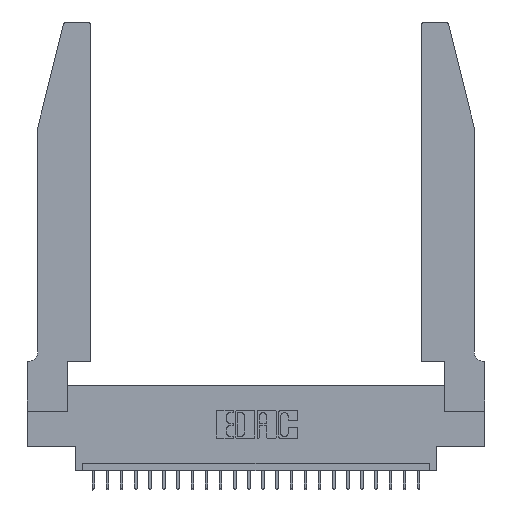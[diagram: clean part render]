
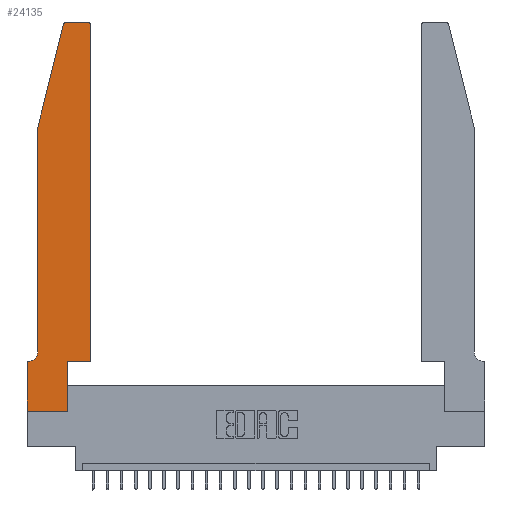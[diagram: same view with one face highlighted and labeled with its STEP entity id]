
A CAD part, top view. The second image highlights one B-rep face of the part: STEP entity #24135.
In plain terms, the highlighted planar face has unit normal (0, 0, 1).
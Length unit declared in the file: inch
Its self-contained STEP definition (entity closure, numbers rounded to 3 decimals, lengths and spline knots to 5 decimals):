
#14 = CARTESIAN_POINT ( 'NONE',  ( 0.4505, 0.35, 0.37 ) ) ;
#51 = AXIS2_PLACEMENT_3D ( 'NONE', #10371, #716, #18200 ) ;
#191 = ORIENTED_EDGE ( 'NONE', *, *, #12260, .T. ) ;
#641 = LINE ( 'NONE', #16233, #10763 ) ;
#716 = DIRECTION ( 'NONE',  ( 0., 0., 1. ) ) ;
#1114 = PLANE ( 'NONE',  #5578 ) ;
#1392 = CARTESIAN_POINT ( 'NONE',  ( 0.0755, 0.35, 0.37 ) ) ;
#1571 = VERTEX_POINT ( 'NONE', #12350 ) ;
#2977 = CARTESIAN_POINT ( 'NONE',  ( 0.0755, 2., 0.37 ) ) ;
#3341 = CARTESIAN_POINT ( 'NONE',  ( 0.0055, 0.42, 0.37 ) ) ;
#3713 = DIRECTION ( 'NONE',  ( -1., 0., 0. ) ) ;
#4016 = ORIENTED_EDGE ( 'NONE', *, *, #24221, .T. ) ;
#4251 = CARTESIAN_POINT ( 'NONE',  ( 0.0755, 2., 0.37 ) ) ;
#4422 = EDGE_CURVE ( 'NONE', #24892, #13779, #7336, .T. ) ;
#4472 = EDGE_CURVE ( 'NONE', #12103, #1571, #8164, .T. ) ;
#5578 = AXIS2_PLACEMENT_3D ( 'NONE', #16710, #6693, #14515 ) ;
#5741 = ORIENTED_EDGE ( 'NONE', *, *, #10918, .T. ) ;
#6001 = CARTESIAN_POINT ( 'NONE',  ( 0.4205, 2.75, 0.37 ) ) ;
#6155 = CARTESIAN_POINT ( 'NONE',  ( 0.2865, 0., 0.37 ) ) ;
#6693 = DIRECTION ( 'NONE',  ( 0., 0., 1. ) ) ;
#6785 = CARTESIAN_POINT ( 'NONE',  ( 0.4505, 0.35, 0.37 ) ) ;
#7231 = DIRECTION ( 'NONE',  ( 0., 1., 0. ) ) ;
#7336 = CIRCLE ( 'NONE', #22119, 0.07 ) ;
#7711 = CARTESIAN_POINT ( 'NONE',  ( 0.4505, 2.72, 0.37 ) ) ;
#8164 = CIRCLE ( 'NONE', #14316, 0.03 ) ;
#8237 = VERTEX_POINT ( 'NONE', #14681 ) ;
#8487 = VECTOR ( 'NONE', #16945, 39.37008 ) ;
#8512 = DIRECTION ( 'NONE',  ( 0., -1., 0. ) ) ;
#8934 = DIRECTION ( 'NONE',  ( 0., 0., 1. ) ) ;
#9115 = FACE_OUTER_BOUND ( 'NONE', #23771, .T. ) ;
#9247 = CARTESIAN_POINT ( 'NONE',  ( 0.2605, 2.75, 0.37 ) ) ;
#9579 = VECTOR ( 'NONE', #3713, 39.37008 ) ;
#9839 = LINE ( 'NONE', #14, #10382 ) ;
#10145 = ORIENTED_EDGE ( 'NONE', *, *, #25281, .T. ) ;
#10371 = CARTESIAN_POINT ( 'NONE',  ( 0.4205, 2.72, 0.37 ) ) ;
#10382 = VECTOR ( 'NONE', #17653, 39.37008 ) ;
#10714 = LINE ( 'NONE', #2977, #22057 ) ;
#10716 = VERTEX_POINT ( 'NONE', #6001 ) ;
#10763 = VECTOR ( 'NONE', #8512, 39.37008 ) ;
#10916 = VECTOR ( 'NONE', #15660, 39.37008 ) ;
#10918 = EDGE_CURVE ( 'NONE', #21798, #10716, #20173, .T. ) ;
#11150 = LINE ( 'NONE', #9247, #20796 ) ;
#11857 = LINE ( 'NONE', #19698, #20212 ) ;
#12103 = VERTEX_POINT ( 'NONE', #17873 ) ;
#12260 = EDGE_CURVE ( 'NONE', #17169, #13302, #641, .T. ) ;
#12350 = CARTESIAN_POINT ( 'NONE',  ( 0.25487, 2.72718, 0.37 ) ) ;
#13122 = VERTEX_POINT ( 'NONE', #24740 ) ;
#13290 = ORIENTED_EDGE ( 'NONE', *, *, #24005, .T. ) ;
#13302 = VERTEX_POINT ( 'NONE', #17529 ) ;
#13452 = ORIENTED_EDGE ( 'NONE', *, *, #4422, .T. ) ;
#13779 = VERTEX_POINT ( 'NONE', #13993 ) ;
#13993 = CARTESIAN_POINT ( 'NONE',  ( 0.0055, 0.35, 0.37 ) ) ;
#14316 = AXIS2_PLACEMENT_3D ( 'NONE', #17143, #8934, #24607 ) ;
#14515 = DIRECTION ( 'NONE',  ( 1., 0., 0. ) ) ;
#14681 = CARTESIAN_POINT ( 'NONE',  ( 0.0755, 2., 0.37 ) ) ;
#14819 = DIRECTION ( 'NONE',  ( -1., 0., 0. ) ) ;
#14838 = CARTESIAN_POINT ( 'NONE',  ( 0., 0.35, 0.37 ) ) ;
#14887 = VECTOR ( 'NONE', #7231, 39.37008 ) ;
#15130 = LINE ( 'NONE', #15531, #10916 ) ;
#15531 = CARTESIAN_POINT ( 'NONE',  ( 0.4505, 0.35, 0.37 ) ) ;
#15660 = DIRECTION ( 'NONE',  ( 0., 1., 0. ) ) ;
#16123 = DIRECTION ( 'NONE',  ( 1., 0., 0. ) ) ;
#16233 = CARTESIAN_POINT ( 'NONE',  ( 0., 0., 0.37 ) ) ;
#16710 = CARTESIAN_POINT ( 'NONE',  ( 0., 0.35, 0.37 ) ) ;
#16945 = DIRECTION ( 'NONE',  ( -0.239, -0.971, 0. ) ) ;
#17143 = CARTESIAN_POINT ( 'NONE',  ( 0.284, 2.72, 0.37 ) ) ;
#17169 = VERTEX_POINT ( 'NONE', #14838 ) ;
#17193 = ORIENTED_EDGE ( 'NONE', *, *, #4472, .T. ) ;
#17529 = CARTESIAN_POINT ( 'NONE',  ( 0., 0., 0.37 ) ) ;
#17653 = DIRECTION ( 'NONE',  ( 1., 0., 0. ) ) ;
#17873 = CARTESIAN_POINT ( 'NONE',  ( 0.284, 2.75, 0.37 ) ) ;
#18200 = DIRECTION ( 'NONE',  ( 1., 0., 0. ) ) ;
#18670 = EDGE_CURVE ( 'NONE', #21903, #13122, #24849, .T. ) ;
#18711 = ORIENTED_EDGE ( 'NONE', *, *, #24792, .T. ) ;
#18784 = CARTESIAN_POINT ( 'NONE',  ( 0.0755, 0.42, 0.37 ) ) ;
#18894 = CARTESIAN_POINT ( 'NONE',  ( 0.2865, 0.35, 0.37 ) ) ;
#18978 = DIRECTION ( 'NONE',  ( -1., 0., 0. ) ) ;
#19200 = VERTEX_POINT ( 'NONE', #6785 ) ;
#19698 = CARTESIAN_POINT ( 'NONE',  ( 0., 0., 0.37 ) ) ;
#19772 = EDGE_CURVE ( 'NONE', #13122, #19200, #9839, .T. ) ;
#19911 = EDGE_CURVE ( 'NONE', #13302, #21903, #11857, .T. ) ;
#20173 = CIRCLE ( 'NONE', #51, 0.03 ) ;
#20212 = VECTOR ( 'NONE', #16123, 39.37008 ) ;
#20252 = EDGE_CURVE ( 'NONE', #13779, #17169, #25220, .T. ) ;
#20796 = VECTOR ( 'NONE', #18978, 39.37008 ) ;
#20840 = DIRECTION ( 'NONE',  ( 0., 0., -1. ) ) ;
#21798 = VERTEX_POINT ( 'NONE', #7711 ) ;
#21863 = LINE ( 'NONE', #4251, #8487 ) ;
#21903 = VERTEX_POINT ( 'NONE', #6155 ) ;
#22057 = VECTOR ( 'NONE', #24257, 39.37008 ) ;
#22119 = AXIS2_PLACEMENT_3D ( 'NONE', #3341, #20840, #14819 ) ;
#22327 = ORIENTED_EDGE ( 'NONE', *, *, #20252, .T. ) ;
#22811 = ORIENTED_EDGE ( 'NONE', *, *, #19911, .T. ) ;
#23490 = ORIENTED_EDGE ( 'NONE', *, *, #19772, .T. ) ;
#23771 = EDGE_LOOP ( 'NONE', ( #10145, #17193, #13290, #18711, #13452, #22327, #191, #22811, #24438, #23490, #4016, #5741 ) ) ;
#24005 = EDGE_CURVE ( 'NONE', #1571, #8237, #21863, .T. ) ;
#24135 = ADVANCED_FACE ( 'NONE', ( #9115 ), #1114, .T. ) ;
#24221 = EDGE_CURVE ( 'NONE', #19200, #21798, #15130, .T. ) ;
#24257 = DIRECTION ( 'NONE',  ( 0., -1., 0. ) ) ;
#24438 = ORIENTED_EDGE ( 'NONE', *, *, #18670, .T. ) ;
#24607 = DIRECTION ( 'NONE',  ( 1., 0., 0. ) ) ;
#24740 = CARTESIAN_POINT ( 'NONE',  ( 0.2865, 0.35, 0.37 ) ) ;
#24792 = EDGE_CURVE ( 'NONE', #8237, #24892, #10714, .T. ) ;
#24849 = LINE ( 'NONE', #18894, #14887 ) ;
#24892 = VERTEX_POINT ( 'NONE', #18784 ) ;
#25220 = LINE ( 'NONE', #1392, #9579 ) ;
#25281 = EDGE_CURVE ( 'NONE', #10716, #12103, #11150, .T. ) ;
